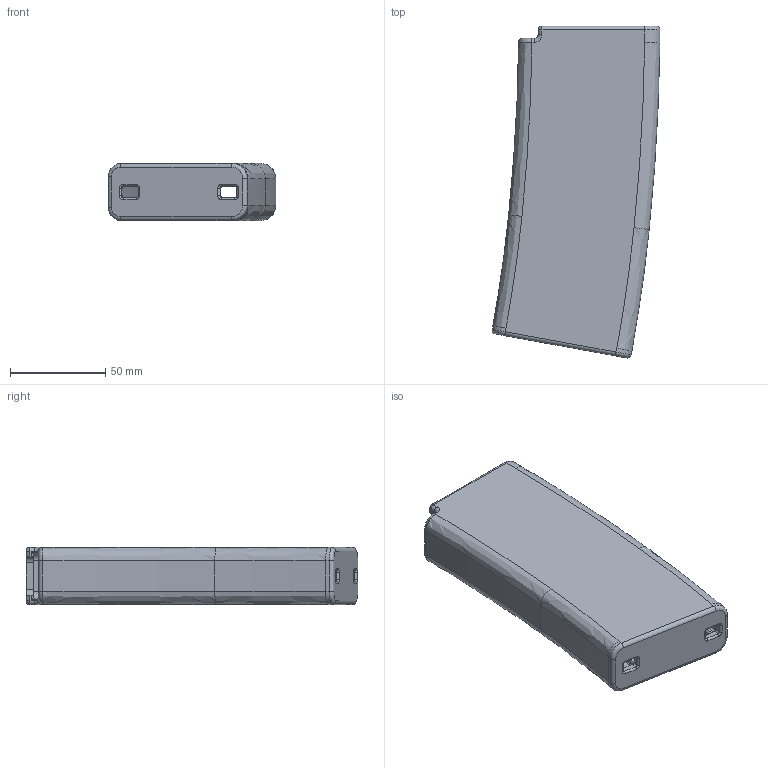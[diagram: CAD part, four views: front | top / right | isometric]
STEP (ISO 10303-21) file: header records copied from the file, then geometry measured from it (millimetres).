
FILE_DESCRIPTION(/* description */ (''),/* implementation_level */ '2;1');
FILE_NAME(/* name */ 'adb5d526-e4c9-4063-aaee-3deb86a92f40.stp',/* time_stamp */ '2019-04-30T20:32:14-04:00',/* author */ ('suzuki450ltr'),/* organization */ (''),/* preprocessor_version */ 'ST-DEVELOPER v18',/* originating_system */ 'Autodesk Translation Framework v8.2.0.1029',/* authorisation */ '');
FILE_SCHEMA (('AUTOMOTIVE_DESIGN { 1 0 10303 214 3 1 1 }'));
Length unit declared in the file: millimetre
Products named in the file (1): Lancer 10RD Mag Extension
Bounding box: 87.88 x 173.83 x 29.9 mm (x, y, z)
Volume: 178712.7 mm3; surface area: 63434.4 mm2
Topology: 1 solids, 1 shells, 266 faces, 641 edges, 372 vertices
Faces by surface type: cylinder 104, bspline 72, plane 48, torus 28, cone 10, sphere 4
Full cylindrical faces by diameter (mm): 3 x1
Entity records: 9391 total; most frequent: CARTESIAN_POINT 3411, ORIENTED_EDGE 1274, DIRECTION 1257, EDGE_CURVE 637, AXIS2_PLACEMENT_3D 507, VERTEX_POINT 372, CIRCLE 304, EDGE_LOOP 269
